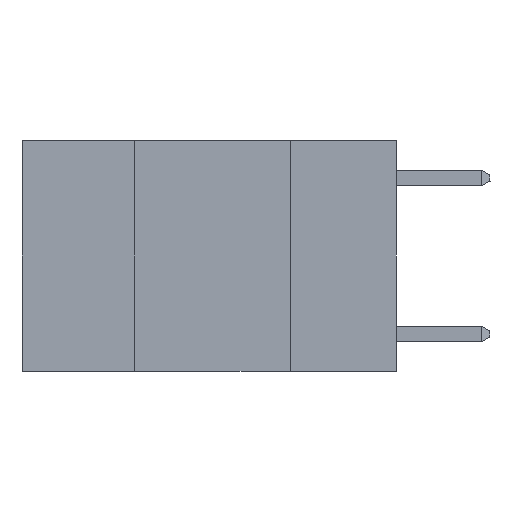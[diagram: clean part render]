
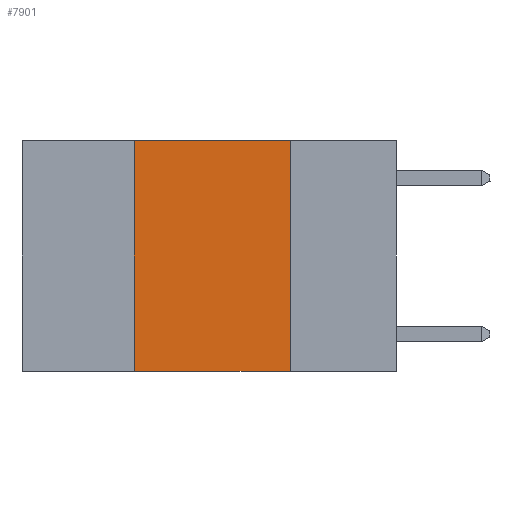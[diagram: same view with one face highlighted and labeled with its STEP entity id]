
A CAD part, left-side view. The second image highlights one B-rep face of the part: STEP entity #7901.
In plain terms, the highlighted planar face has unit normal (-1, 0, 0).
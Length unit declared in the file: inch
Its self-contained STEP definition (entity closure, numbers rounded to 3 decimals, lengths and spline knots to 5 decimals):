
#133 = DIRECTION ( 'NONE',  ( 0., 0., -1. ) ) ;
#471 = ORIENTED_EDGE ( 'NONE', *, *, #5238, .F. ) ;
#477 = EDGE_CURVE ( 'NONE', #3879, #4947, #8671, .T. ) ;
#498 = ORIENTED_EDGE ( 'NONE', *, *, #3196, .F. ) ;
#534 = ORIENTED_EDGE ( 'NONE', *, *, #1353, .F. ) ;
#644 = ORIENTED_EDGE ( 'NONE', *, *, #477, .T. ) ;
#841 = LINE ( 'NONE', #1921, #8455 ) ;
#1353 = EDGE_CURVE ( 'NONE', #1680, #4922, #841, .T. ) ;
#1645 = CARTESIAN_POINT ( 'NONE',  ( 0., 0.17, 0. ) ) ;
#1680 = VERTEX_POINT ( 'NONE', #6227 ) ;
#1921 = CARTESIAN_POINT ( 'NONE',  ( 0., 0.6, 0. ) ) ;
#2228 = AXIS2_PLACEMENT_3D ( 'NONE', #8716, #4656, #133 ) ;
#2501 = CARTESIAN_POINT ( 'NONE',  ( 0., 0.6, -0.37 ) ) ;
#3097 = VECTOR ( 'NONE', #9011, 39.37008 ) ;
#3196 = EDGE_CURVE ( 'NONE', #4922, #4947, #5260, .T. ) ;
#3512 = DIRECTION ( 'NONE',  ( 0., 0., 1. ) ) ;
#3879 = VERTEX_POINT ( 'NONE', #4846 ) ;
#4656 = DIRECTION ( 'NONE',  ( 1., 0., 0. ) ) ;
#4720 = LINE ( 'NONE', #8350, #6138 ) ;
#4846 = CARTESIAN_POINT ( 'NONE',  ( 0., 0.42, -0.37 ) ) ;
#4922 = VERTEX_POINT ( 'NONE', #1645 ) ;
#4947 = VERTEX_POINT ( 'NONE', #5390 ) ;
#5238 = EDGE_CURVE ( 'NONE', #3879, #1680, #4720, .T. ) ;
#5260 = LINE ( 'NONE', #7605, #6222 ) ;
#5390 = CARTESIAN_POINT ( 'NONE',  ( 0., 0.17, -0.37 ) ) ;
#6138 = VECTOR ( 'NONE', #3512, 39.37008 ) ;
#6222 = VECTOR ( 'NONE', #7871, 39.37008 ) ;
#6227 = CARTESIAN_POINT ( 'NONE',  ( 0., 0.42, 0. ) ) ;
#7227 = EDGE_LOOP ( 'NONE', ( #498, #534, #471, #644 ) ) ;
#7384 = PLANE ( 'NONE',  #2228 ) ;
#7605 = CARTESIAN_POINT ( 'NONE',  ( 0., 0.17, 0. ) ) ;
#7871 = DIRECTION ( 'NONE',  ( 0., 0., -1. ) ) ;
#7901 = ADVANCED_FACE ( 'NONE', ( #8694 ), #7384, .F. ) ;
#8350 = CARTESIAN_POINT ( 'NONE',  ( 0., 0.42, 0. ) ) ;
#8447 = DIRECTION ( 'NONE',  ( 0., -1., 0. ) ) ;
#8455 = VECTOR ( 'NONE', #8447, 39.37008 ) ;
#8671 = LINE ( 'NONE', #2501, #3097 ) ;
#8694 = FACE_OUTER_BOUND ( 'NONE', #7227, .T. ) ;
#8716 = CARTESIAN_POINT ( 'NONE',  ( 0., 0.6, 0. ) ) ;
#9011 = DIRECTION ( 'NONE',  ( 0., -1., 0. ) ) ;
